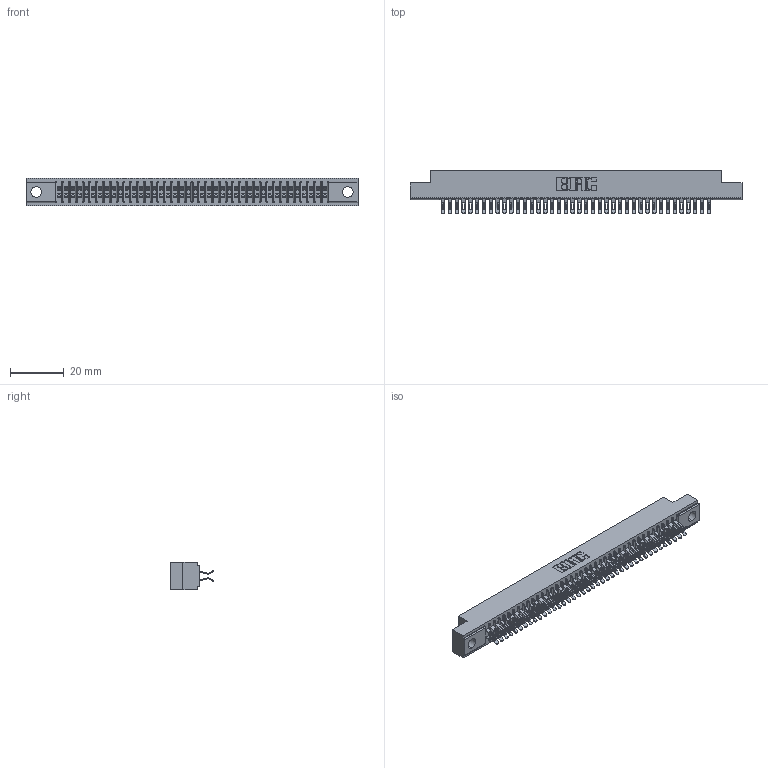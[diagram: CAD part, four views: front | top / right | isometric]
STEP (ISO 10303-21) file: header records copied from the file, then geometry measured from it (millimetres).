
FILE_DESCRIPTION (( 'STEP AP203' ), '1' );
FILE_NAME ('391-080-555-204.STEP', '2018-08-09T15:44:35', ( '' ), ( '' ), 'SwSTEP 2.0', 'SolidWorks 2016', '' );
FILE_SCHEMA (( 'CONFIG_CONTROL_DESIGN' ));
Length unit declared in the file: inch
Products named in the file (3): 341 Part_.156 (3.96) Dia Mounting Holes; 341-292-001_341-292-155; 391-080-555-204
Assembly tree (81 placements, depth 2):
  391-080-555-204
    341 Part_.156 (3.96) Dia Mounting Holes
    341-292-001_341-292-155  x80
Bounding box: 123.83 x 16.31 x 10.16 mm (x, y, z)
Volume: 9137.8 mm3; surface area: 16696.9 mm2
Topology: 81 solids, 81 shells, 6370 faces, 19032 edges, 12390 vertices
Faces by surface type: plane 3442, cylinder 2768, sphere 82, torus 78
Entity records: 49563 total; most frequent: CARTESIAN_POINT 8260, ORIENTED_EDGE 8196, DIRECTION 8000, EDGE_CURVE 4098, LINE 3300, VECTOR 3300, VERTEX_POINT 2594, AXIS2_PLACEMENT_3D 2350
